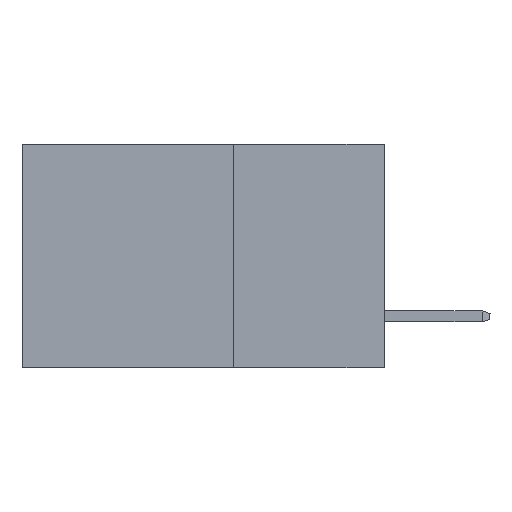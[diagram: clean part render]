
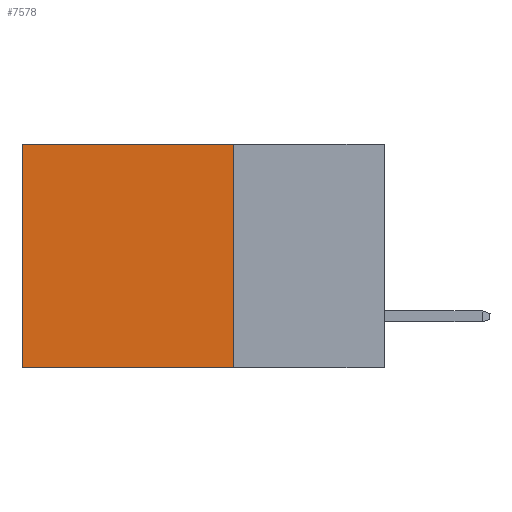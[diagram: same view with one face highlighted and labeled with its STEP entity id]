
A CAD part, left-side view. The second image highlights one B-rep face of the part: STEP entity #7578.
In plain terms, the highlighted planar face has unit normal (-1, 0, 0).
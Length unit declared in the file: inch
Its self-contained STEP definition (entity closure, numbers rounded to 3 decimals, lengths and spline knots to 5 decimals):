
#345 = CARTESIAN_POINT ( 'NONE',  ( 0.2615, 0.25, 0. ) ) ;
#484 = LINE ( 'NONE', #345, #6782 ) ;
#1213 = VERTEX_POINT ( 'NONE', #4024 ) ;
#1310 = CARTESIAN_POINT ( 'NONE',  ( 0.2615, 0.6, -0.37 ) ) ;
#1622 = DIRECTION ( 'NONE',  ( 0., 1., 0. ) ) ;
#1876 = EDGE_LOOP ( 'NONE', ( #3570, #3372, #9686, #3256 ) ) ;
#2058 = CARTESIAN_POINT ( 'NONE',  ( 0.2615, 0.6, -0.37 ) ) ;
#2116 = EDGE_CURVE ( 'NONE', #3799, #11558, #6302, .T. ) ;
#2392 = DIRECTION ( 'NONE',  ( 0., 0., -1. ) ) ;
#2781 = DIRECTION ( 'NONE',  ( 0., 0., -1. ) ) ;
#3256 = ORIENTED_EDGE ( 'NONE', *, *, #10578, .T. ) ;
#3281 = LINE ( 'NONE', #12517, #10226 ) ;
#3372 = ORIENTED_EDGE ( 'NONE', *, *, #9031, .F. ) ;
#3570 = ORIENTED_EDGE ( 'NONE', *, *, #2116, .T. ) ;
#3799 = VERTEX_POINT ( 'NONE', #5480 ) ;
#4024 = CARTESIAN_POINT ( 'NONE',  ( 0.2615, 0.25, 0. ) ) ;
#4571 = CARTESIAN_POINT ( 'NONE',  ( 0.2615, 0.25, -0.37 ) ) ;
#4781 = VERTEX_POINT ( 'NONE', #10949 ) ;
#5024 = LINE ( 'NONE', #13184, #10426 ) ;
#5480 = CARTESIAN_POINT ( 'NONE',  ( 0.2615, 0.6, 0. ) ) ;
#6024 = VECTOR ( 'NONE', #6099, 39.37008 ) ;
#6099 = DIRECTION ( 'NONE',  ( 0., 0., -1. ) ) ;
#6302 = LINE ( 'NONE', #2058, #6024 ) ;
#6782 = VECTOR ( 'NONE', #1622, 39.37008 ) ;
#7578 = ADVANCED_FACE ( 'NONE', ( #10717 ), #12002, .F. ) ;
#8033 = EDGE_CURVE ( 'NONE', #1213, #4781, #5024, .T. ) ;
#8471 = AXIS2_PLACEMENT_3D ( 'NONE', #4571, #12735, #2392 ) ;
#9031 = EDGE_CURVE ( 'NONE', #4781, #11558, #3281, .T. ) ;
#9554 = DIRECTION ( 'NONE',  ( 0., 1., 0. ) ) ;
#9686 = ORIENTED_EDGE ( 'NONE', *, *, #8033, .F. ) ;
#10226 = VECTOR ( 'NONE', #9554, 39.37008 ) ;
#10426 = VECTOR ( 'NONE', #2781, 39.37008 ) ;
#10578 = EDGE_CURVE ( 'NONE', #1213, #3799, #484, .T. ) ;
#10717 = FACE_OUTER_BOUND ( 'NONE', #1876, .T. ) ;
#10949 = CARTESIAN_POINT ( 'NONE',  ( 0.2615, 0.25, -0.37 ) ) ;
#11558 = VERTEX_POINT ( 'NONE', #1310 ) ;
#12002 = PLANE ( 'NONE',  #8471 ) ;
#12517 = CARTESIAN_POINT ( 'NONE',  ( 0.2615, 0.25, -0.37 ) ) ;
#12735 = DIRECTION ( 'NONE',  ( 1., 0., 0. ) ) ;
#13184 = CARTESIAN_POINT ( 'NONE',  ( 0.2615, 0.25, -0.37 ) ) ;
